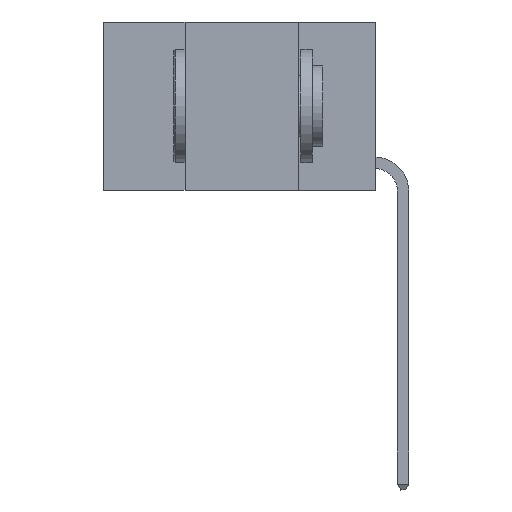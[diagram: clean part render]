
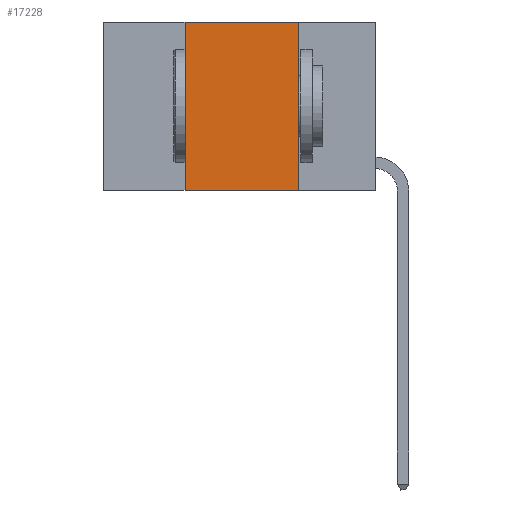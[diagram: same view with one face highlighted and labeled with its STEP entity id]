
A CAD part, left-side view. The second image highlights one B-rep face of the part: STEP entity #17228.
In plain terms, the highlighted planar face has unit normal (-1, 0, 0).
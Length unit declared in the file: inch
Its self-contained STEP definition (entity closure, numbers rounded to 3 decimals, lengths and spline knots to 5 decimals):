
#1516 = EDGE_LOOP ( 'NONE', ( #11565, #24698, #10321, #9707 ) ) ;
#1569 = LINE ( 'NONE', #19735, #16101 ) ;
#1776 = VERTEX_POINT ( 'NONE', #19058 ) ;
#1864 = CARTESIAN_POINT ( 'NONE',  ( 0., 0.17, 0. ) ) ;
#4122 = DIRECTION ( 'NONE',  ( 0., 0., 1. ) ) ;
#4911 = VECTOR ( 'NONE', #17075, 39.37008 ) ;
#6740 = VERTEX_POINT ( 'NONE', #23581 ) ;
#6951 = EDGE_CURVE ( 'NONE', #17530, #14955, #1569, .T. ) ;
#8640 = FACE_OUTER_BOUND ( 'NONE', #1516, .T. ) ;
#9663 = EDGE_CURVE ( 'NONE', #17530, #6740, #16191, .T. ) ;
#9707 = ORIENTED_EDGE ( 'NONE', *, *, #9663, .T. ) ;
#10321 = ORIENTED_EDGE ( 'NONE', *, *, #6951, .F. ) ;
#10761 = DIRECTION ( 'NONE',  ( 1., 0., 0. ) ) ;
#11164 = VECTOR ( 'NONE', #16427, 39.37008 ) ;
#11565 = ORIENTED_EDGE ( 'NONE', *, *, #20694, .F. ) ;
#11914 = LINE ( 'NONE', #24756, #11164 ) ;
#14955 = VERTEX_POINT ( 'NONE', #26914 ) ;
#16101 = VECTOR ( 'NONE', #4122, 39.37008 ) ;
#16191 = LINE ( 'NONE', #18156, #27413 ) ;
#16363 = LINE ( 'NONE', #1864, #4911 ) ;
#16427 = DIRECTION ( 'NONE',  ( 0., -1., 0. ) ) ;
#17075 = DIRECTION ( 'NONE',  ( 0., 0., -1. ) ) ;
#17228 = ADVANCED_FACE ( 'NONE', ( #8640 ), #25567, .F. ) ;
#17530 = VERTEX_POINT ( 'NONE', #18058 ) ;
#18058 = CARTESIAN_POINT ( 'NONE',  ( 0., 0.42, -0.37 ) ) ;
#18156 = CARTESIAN_POINT ( 'NONE',  ( 0., 0.6, -0.37 ) ) ;
#19058 = CARTESIAN_POINT ( 'NONE',  ( 0., 0.17, 0. ) ) ;
#19627 = CARTESIAN_POINT ( 'NONE',  ( 0., 0.6, 0. ) ) ;
#19735 = CARTESIAN_POINT ( 'NONE',  ( 0., 0.42, 0. ) ) ;
#19779 = EDGE_CURVE ( 'NONE', #14955, #1776, #11914, .T. ) ;
#20283 = DIRECTION ( 'NONE',  ( 0., -1., 0. ) ) ;
#20694 = EDGE_CURVE ( 'NONE', #1776, #6740, #16363, .T. ) ;
#23581 = CARTESIAN_POINT ( 'NONE',  ( 0., 0.17, -0.37 ) ) ;
#24698 = ORIENTED_EDGE ( 'NONE', *, *, #19779, .F. ) ;
#24756 = CARTESIAN_POINT ( 'NONE',  ( 0., 0.6, 0. ) ) ;
#25567 = PLANE ( 'NONE',  #25619 ) ;
#25619 = AXIS2_PLACEMENT_3D ( 'NONE', #19627, #10761, #27813 ) ;
#26914 = CARTESIAN_POINT ( 'NONE',  ( 0., 0.42, 0. ) ) ;
#27413 = VECTOR ( 'NONE', #20283, 39.37008 ) ;
#27813 = DIRECTION ( 'NONE',  ( 0., 0., -1. ) ) ;
